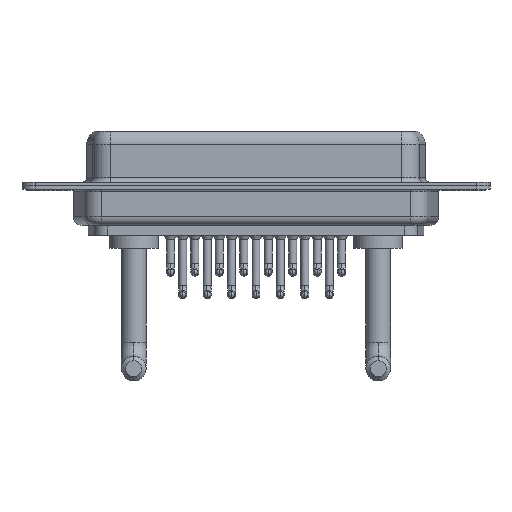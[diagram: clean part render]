
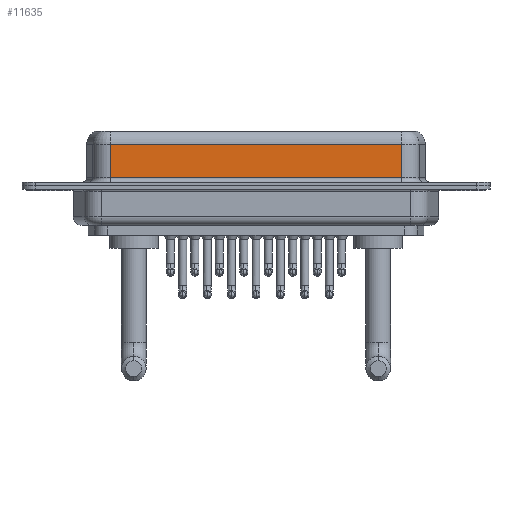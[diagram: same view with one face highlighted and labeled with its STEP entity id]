
A CAD part, front view. The second image highlights one B-rep face of the part: STEP entity #11635.
In plain terms, the highlighted planar face has unit normal (0, -1, 0).
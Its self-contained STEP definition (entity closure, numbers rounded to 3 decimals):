
#91 = DIRECTION ( 'NONE',  ( 0., 1., 0. ) ) ;
#454 = CARTESIAN_POINT ( 'NONE',  ( 7.013, -3.95, 0.9 ) ) ;
#780 = VECTOR ( 'NONE', #13727, 1000. ) ;
#999 = LINE ( 'NONE', #2366, #6029 ) ;
#2189 = EDGE_CURVE ( 'NONE', #18535, #13691, #3027, .T. ) ;
#2366 = CARTESIAN_POINT ( 'NONE',  ( 7.013, -3.95, 6.4 ) ) ;
#2656 = EDGE_CURVE ( 'NONE', #18535, #14028, #6088, .T. ) ;
#2710 = CARTESIAN_POINT ( 'NONE',  ( 40.037, -3.95, 4.65 ) ) ;
#3027 = LINE ( 'NONE', #9204, #780 ) ;
#3720 = ORIENTED_EDGE ( 'NONE', *, *, #2656, .T. ) ;
#4119 = ORIENTED_EDGE ( 'NONE', *, *, #8940, .T. ) ;
#6029 = VECTOR ( 'NONE', #8264, 1000. ) ;
#6088 = LINE ( 'NONE', #16666, #11191 ) ;
#7285 = ORIENTED_EDGE ( 'NONE', *, *, #2189, .F. ) ;
#7778 = LINE ( 'NONE', #13659, #15258 ) ;
#7989 = DIRECTION ( 'NONE',  ( -1., 0., 0. ) ) ;
#7996 = CARTESIAN_POINT ( 'NONE',  ( 7.013, -3.95, 4.65 ) ) ;
#8264 = DIRECTION ( 'NONE',  ( 0., 0., -1. ) ) ;
#8760 = EDGE_CURVE ( 'NONE', #10667, #13691, #7778, .T. ) ;
#8940 = EDGE_CURVE ( 'NONE', #14028, #10667, #999, .T. ) ;
#9204 = CARTESIAN_POINT ( 'NONE',  ( 40.037, -3.95, 6.4 ) ) ;
#9626 = ORIENTED_EDGE ( 'NONE', *, *, #8760, .T. ) ;
#10144 = CARTESIAN_POINT ( 'NONE',  ( 40.037, -3.95, 6.4 ) ) ;
#10667 = VERTEX_POINT ( 'NONE', #454 ) ;
#11191 = VECTOR ( 'NONE', #7989, 1000. ) ;
#11635 = ADVANCED_FACE ( 'NONE', ( #17559 ), #17361, .F. ) ;
#11641 = CARTESIAN_POINT ( 'NONE',  ( 40.037, -3.95, 0.9 ) ) ;
#13493 = AXIS2_PLACEMENT_3D ( 'NONE', #10144, #91, #16010 ) ;
#13659 = CARTESIAN_POINT ( 'NONE',  ( 40.037, -3.95, 0.9 ) ) ;
#13691 = VERTEX_POINT ( 'NONE', #11641 ) ;
#13727 = DIRECTION ( 'NONE',  ( 0., 0., -1. ) ) ;
#14028 = VERTEX_POINT ( 'NONE', #7996 ) ;
#15258 = VECTOR ( 'NONE', #18090, 1000. ) ;
#16010 = DIRECTION ( 'NONE',  ( 0., 0., 1. ) ) ;
#16666 = CARTESIAN_POINT ( 'NONE',  ( 40.037, -3.95, 4.65 ) ) ;
#17361 = PLANE ( 'NONE',  #13493 ) ;
#17559 = FACE_OUTER_BOUND ( 'NONE', #17738, .T. ) ;
#17738 = EDGE_LOOP ( 'NONE', ( #7285, #3720, #4119, #9626 ) ) ;
#18090 = DIRECTION ( 'NONE',  ( 1., 0., 0. ) ) ;
#18535 = VERTEX_POINT ( 'NONE', #2710 ) ;
